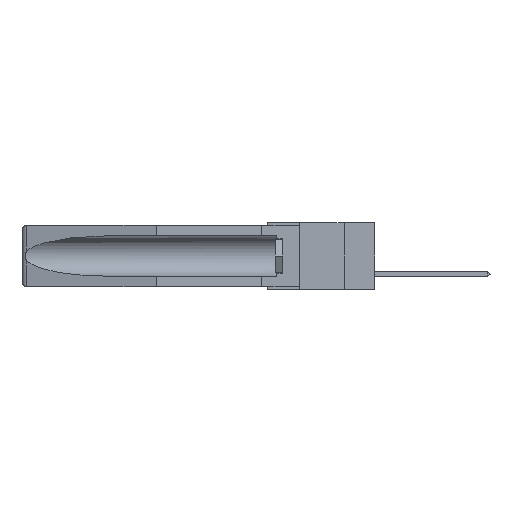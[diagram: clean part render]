
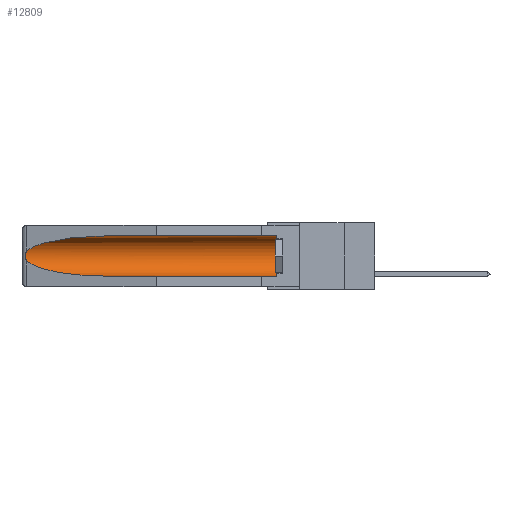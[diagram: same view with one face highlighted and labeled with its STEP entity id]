
A CAD part, left-side view. The second image highlights one B-rep face of the part: STEP entity #12809.
In plain terms, the highlighted cylindrical face has radius 2.857 mm (diameter 5.715 mm), a partial arc.
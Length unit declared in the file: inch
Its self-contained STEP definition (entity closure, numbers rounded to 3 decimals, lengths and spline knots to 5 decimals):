
#16 = CARTESIAN_POINT ( 'NONE',  ( 0.25451, 1.48313, -0.09465 ) ) ;
#211 = CARTESIAN_POINT ( 'NONE',  ( 0.21114, 1.30732, -0.284 ) ) ;
#758 = VECTOR ( 'NONE', #13659, 39.37008 ) ;
#1503 = CARTESIAN_POINT ( 'NONE',  ( 0.155, -0.30754, -0.284 ) ) ;
#1812 = CARTESIAN_POINT ( 'NONE',  ( 0.26537, 1.52718, -0.14972 ) ) ;
#2521 = CARTESIAN_POINT ( 'NONE',  ( 0.155, 0.126, -0.284 ) ) ;
#2829 = EDGE_LOOP ( 'NONE', ( #19181, #16275, #9391, #16986, #19955, #13255 ) ) ;
#3532 = DIRECTION ( 'NONE',  ( 0., 0., 1. ) ) ;
#3804 = CIRCLE ( 'NONE', #20045, 0.1125 ) ;
#3877 = CARTESIAN_POINT ( 'NONE',  ( 0.25451, 1.48313, -0.24835 ) ) ;
#3997 = EDGE_CURVE ( 'NONE', #18371, #14046, #3804, .T. ) ;
#4235 =( BOUNDED_CURVE ( )  B_SPLINE_CURVE ( 3, ( #12381, #3877, #211, #15818 ),
 .UNSPECIFIED., .F., .F. ) 
 B_SPLINE_CURVE_WITH_KNOTS ( ( 4, 4 ),
 ( 0.1948, 1.5708 ),
 .UNSPECIFIED. ) 
 CURVE ( )  GEOMETRIC_REPRESENTATION_ITEM ( )  RATIONAL_B_SPLINE_CURVE ( ( 1., 0.848, 0.848, 1. ) ) 
 REPRESENTATION_ITEM ( '' )  );
#4916 = CARTESIAN_POINT ( 'NONE',  ( 0.155, 1.07973, -0.284 ) ) ;
#4964 = CARTESIAN_POINT ( 'NONE',  ( 0.26537, 1.52718, -0.14972 ) ) ;
#5308 = CARTESIAN_POINT ( 'NONE',  ( 0.155, 1.07973, -0.059 ) ) ;
#5451 = EDGE_CURVE ( 'NONE', #5742, #9005, #10503, .T. ) ;
#5595 = LINE ( 'NONE', #1503, #19242 ) ;
#5742 = VERTEX_POINT ( 'NONE', #12285 ) ;
#5851 = CARTESIAN_POINT ( 'NONE',  ( 0.2675, 1.53308, -0.17534 ) ) ;
#6155 = CARTESIAN_POINT ( 'NONE',  ( 0.26597, 1.5296, -0.19026 ) ) ;
#6941 = CARTESIAN_POINT ( 'NONE',  ( 0.21114, 1.30732, -0.059 ) ) ;
#6967 = CARTESIAN_POINT ( 'NONE',  ( 0.155, 0.126, -0.059 ) ) ;
#7506 = CARTESIAN_POINT ( 'NONE',  ( 0.26654, 1.53092, -0.15636 ) ) ;
#7574 = VERTEX_POINT ( 'NONE', #10254 ) ;
#7881 = CARTESIAN_POINT ( 'NONE',  ( 0.26537, 1.52718, -0.19328 ) ) ;
#9005 = VERTEX_POINT ( 'NONE', #4964 ) ;
#9151 = CARTESIAN_POINT ( 'NONE',  ( 0.26537, 1.52718, -0.14972 ) ) ;
#9304 = LINE ( 'NONE', #20403, #758 ) ;
#9391 = ORIENTED_EDGE ( 'NONE', *, *, #16957, .T. ) ;
#10254 = CARTESIAN_POINT ( 'NONE',  ( 0.26537, 1.52718, -0.19328 ) ) ;
#10503 =( BOUNDED_CURVE ( )  B_SPLINE_CURVE ( 3, ( #5308, #6941, #16, #1812 ),
 .UNSPECIFIED., .F., .F. ) 
 B_SPLINE_CURVE_WITH_KNOTS ( ( 4, 4 ),
 ( 4.71239, 6.08839 ),
 .UNSPECIFIED. ) 
 CURVE ( )  GEOMETRIC_REPRESENTATION_ITEM ( )  RATIONAL_B_SPLINE_CURVE ( ( 1., 0.848, 0.848, 1. ) ) 
 REPRESENTATION_ITEM ( '' )  );
#11029 = FACE_OUTER_BOUND ( 'NONE', #2829, .T. ) ;
#12285 = CARTESIAN_POINT ( 'NONE',  ( 0.155, 1.07973, -0.059 ) ) ;
#12381 = CARTESIAN_POINT ( 'NONE',  ( 0.26537, 1.52718, -0.19328 ) ) ;
#12809 = ADVANCED_FACE ( 'NONE', ( #11029 ), #20937, .F. ) ;
#13199 = VERTEX_POINT ( 'NONE', #4916 ) ;
#13255 = ORIENTED_EDGE ( 'NONE', *, *, #20419, .T. ) ;
#13594 = DIRECTION ( 'NONE',  ( 0., 1., 0. ) ) ;
#13659 = DIRECTION ( 'NONE',  ( 0., 1., 0. ) ) ;
#14046 = VERTEX_POINT ( 'NONE', #6967 ) ;
#14396 = CARTESIAN_POINT ( 'NONE',  ( 0.26655, 1.53094, -0.18657 ) ) ;
#14783 = EDGE_CURVE ( 'NONE', #9005, #7574, #16121, .T. ) ;
#15818 = CARTESIAN_POINT ( 'NONE',  ( 0.155, 1.07973, -0.284 ) ) ;
#16121 = B_SPLINE_CURVE_WITH_KNOTS ( 'NONE', 3,
 ( #9151, #21123, #7506, #19694, #16333, #5851, #17822, #14396, #6155, #7881 ),
 .UNSPECIFIED., .F., .F.,
 ( 4, 2, 2, 2, 4 ),
 ( 0., 0.00029, 0.00058, 0.00087, 0.00117 ),
 .UNSPECIFIED. ) ;
#16275 = ORIENTED_EDGE ( 'NONE', *, *, #14783, .T. ) ;
#16333 = CARTESIAN_POINT ( 'NONE',  ( 0.2675, 1.53308, -0.16763 ) ) ;
#16540 = CARTESIAN_POINT ( 'NONE',  ( 0.155, 0.126, -0.1715 ) ) ;
#16957 = EDGE_CURVE ( 'NONE', #7574, #13199, #4235, .T. ) ;
#16986 = ORIENTED_EDGE ( 'NONE', *, *, #22098, .F. ) ;
#17822 = CARTESIAN_POINT ( 'NONE',  ( 0.2673, 1.53269, -0.17917 ) ) ;
#18246 = AXIS2_PLACEMENT_3D ( 'NONE', #22155, #18753, #3532 ) ;
#18371 = VERTEX_POINT ( 'NONE', #2521 ) ;
#18406 = DIRECTION ( 'NONE',  ( 0., 0., 1. ) ) ;
#18753 = DIRECTION ( 'NONE',  ( 0., 1., 0. ) ) ;
#19181 = ORIENTED_EDGE ( 'NONE', *, *, #5451, .T. ) ;
#19242 = VECTOR ( 'NONE', #13594, 39.37008 ) ;
#19694 = CARTESIAN_POINT ( 'NONE',  ( 0.2673, 1.5327, -0.16383 ) ) ;
#19955 = ORIENTED_EDGE ( 'NONE', *, *, #3997, .T. ) ;
#20045 = AXIS2_PLACEMENT_3D ( 'NONE', #16540, #21764, #18406 ) ;
#20403 = CARTESIAN_POINT ( 'NONE',  ( 0.155, -0.30754, -0.059 ) ) ;
#20419 = EDGE_CURVE ( 'NONE', #14046, #5742, #9304, .T. ) ;
#20937 = CYLINDRICAL_SURFACE ( 'NONE', #18246, 0.1125 ) ;
#21123 = CARTESIAN_POINT ( 'NONE',  ( 0.26597, 1.52961, -0.15275 ) ) ;
#21764 = DIRECTION ( 'NONE',  ( 0., -1., 0. ) ) ;
#22098 = EDGE_CURVE ( 'NONE', #18371, #13199, #5595, .T. ) ;
#22155 = CARTESIAN_POINT ( 'NONE',  ( 0.155, -0.30754, -0.1715 ) ) ;
